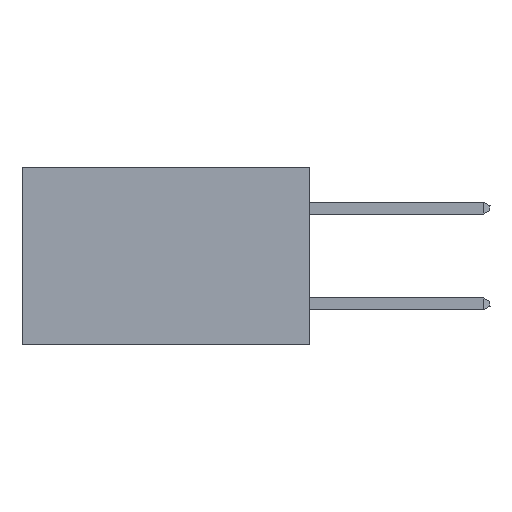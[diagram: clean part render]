
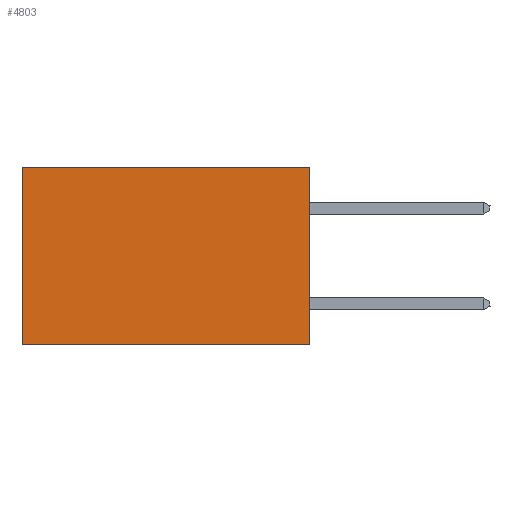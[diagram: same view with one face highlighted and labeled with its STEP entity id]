
A CAD part, left-side view. The second image highlights one B-rep face of the part: STEP entity #4803.
In plain terms, the highlighted planar face has unit normal (-1, 0, 0).
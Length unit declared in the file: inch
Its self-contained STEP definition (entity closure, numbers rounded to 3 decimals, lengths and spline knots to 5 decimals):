
#2504 = CARTESIAN_POINT ( 'NONE',  ( 0.2875, 0.6, 0. ) ) ;
#4803 = ADVANCED_FACE ( 'NONE', ( #18317 ), #26028, .F. ) ;
#5620 = CARTESIAN_POINT ( 'NONE',  ( 0.2875, 0., -0.37 ) ) ;
#5817 = EDGE_CURVE ( 'NONE', #28105, #6464, #9602, .T. ) ;
#5990 = ORIENTED_EDGE ( 'NONE', *, *, #31320, .F. ) ;
#6023 = CARTESIAN_POINT ( 'NONE',  ( 0.2875, 0., 0. ) ) ;
#6318 = LINE ( 'NONE', #12301, #11900 ) ;
#6464 = VERTEX_POINT ( 'NONE', #26173 ) ;
#7907 = AXIS2_PLACEMENT_3D ( 'NONE', #31016, #18511, #26137 ) ;
#8675 = ORIENTED_EDGE ( 'NONE', *, *, #11371, .T. ) ;
#9177 = CARTESIAN_POINT ( 'NONE',  ( 0.2875, 0., 0. ) ) ;
#9602 = LINE ( 'NONE', #18459, #15482 ) ;
#10169 = ORIENTED_EDGE ( 'NONE', *, *, #30091, .F. ) ;
#10733 = ORIENTED_EDGE ( 'NONE', *, *, #5817, .T. ) ;
#10805 = LINE ( 'NONE', #9177, #22602 ) ;
#10981 = DIRECTION ( 'NONE',  ( 0., 0., -1. ) ) ;
#10987 = CARTESIAN_POINT ( 'NONE',  ( 0.2875, 0., 0. ) ) ;
#11371 = EDGE_CURVE ( 'NONE', #23515, #28105, #15582, .T. ) ;
#11601 = EDGE_LOOP ( 'NONE', ( #10733, #10169, #5990, #8675 ) ) ;
#11900 = VECTOR ( 'NONE', #15139, 39.37008 ) ;
#12301 = CARTESIAN_POINT ( 'NONE',  ( 0.2875, 0., -0.37 ) ) ;
#15139 = DIRECTION ( 'NONE',  ( 0., 1., 0. ) ) ;
#15482 = VECTOR ( 'NONE', #10981, 39.37008 ) ;
#15582 = LINE ( 'NONE', #6023, #32197 ) ;
#18317 = FACE_OUTER_BOUND ( 'NONE', #11601, .T. ) ;
#18459 = CARTESIAN_POINT ( 'NONE',  ( 0.2875, 0.6, 0. ) ) ;
#18511 = DIRECTION ( 'NONE',  ( 1., 0., 0. ) ) ;
#20899 = DIRECTION ( 'NONE',  ( 0., 1., 0. ) ) ;
#22602 = VECTOR ( 'NONE', #32667, 39.37008 ) ;
#23515 = VERTEX_POINT ( 'NONE', #10987 ) ;
#26028 = PLANE ( 'NONE',  #7907 ) ;
#26137 = DIRECTION ( 'NONE',  ( 0., 0., -1. ) ) ;
#26173 = CARTESIAN_POINT ( 'NONE',  ( 0.2875, 0.6, -0.37 ) ) ;
#26304 = VERTEX_POINT ( 'NONE', #5620 ) ;
#28105 = VERTEX_POINT ( 'NONE', #2504 ) ;
#30091 = EDGE_CURVE ( 'NONE', #26304, #6464, #6318, .T. ) ;
#31016 = CARTESIAN_POINT ( 'NONE',  ( 0.2875, 0., 0. ) ) ;
#31320 = EDGE_CURVE ( 'NONE', #23515, #26304, #10805, .T. ) ;
#32197 = VECTOR ( 'NONE', #20899, 39.37008 ) ;
#32667 = DIRECTION ( 'NONE',  ( 0., 0., -1. ) ) ;
